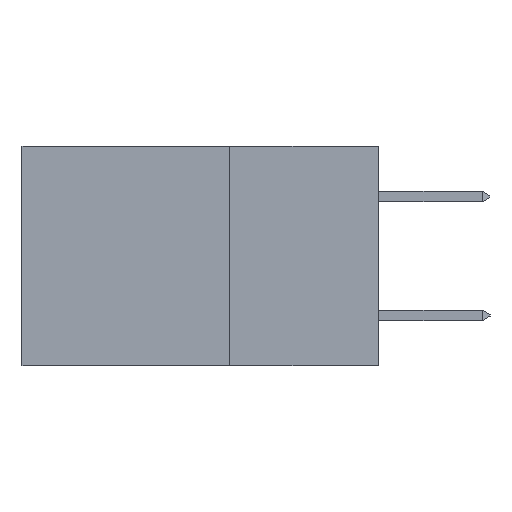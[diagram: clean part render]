
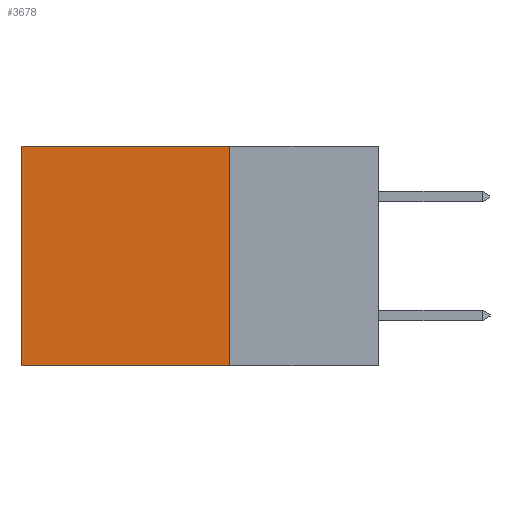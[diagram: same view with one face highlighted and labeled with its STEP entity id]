
A CAD part, left-side view. The second image highlights one B-rep face of the part: STEP entity #3678.
In plain terms, the highlighted planar face has unit normal (-1, 0, 0).
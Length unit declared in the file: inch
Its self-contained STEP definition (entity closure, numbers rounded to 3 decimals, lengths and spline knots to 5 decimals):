
#408 = VERTEX_POINT ( 'NONE', #5674 ) ;
#732 = VERTEX_POINT ( 'NONE', #3483 ) ;
#776 = DIRECTION ( 'NONE',  ( 0., 0., -1. ) ) ;
#1449 = ORIENTED_EDGE ( 'NONE', *, *, #1656, .F. ) ;
#1581 = VECTOR ( 'NONE', #10185, 39.37008 ) ;
#1656 = EDGE_CURVE ( 'NONE', #408, #4252, #3957, .T. ) ;
#1859 = CARTESIAN_POINT ( 'NONE',  ( 0.2615, 0.25, -0.37 ) ) ;
#1880 = VERTEX_POINT ( 'NONE', #9168 ) ;
#1961 = VECTOR ( 'NONE', #7360, 39.37008 ) ;
#2216 = DIRECTION ( 'NONE',  ( 1., 0., 0. ) ) ;
#2349 = EDGE_LOOP ( 'NONE', ( #9094, #3860, #1449, #4312 ) ) ;
#2393 = EDGE_CURVE ( 'NONE', #408, #1880, #5468, .T. ) ;
#3005 = CARTESIAN_POINT ( 'NONE',  ( 0.2615, 0.25, -0.37 ) ) ;
#3154 = FACE_OUTER_BOUND ( 'NONE', #2349, .T. ) ;
#3483 = CARTESIAN_POINT ( 'NONE',  ( 0.2615, 0.6, -0.37 ) ) ;
#3678 = ADVANCED_FACE ( 'NONE', ( #3154 ), #7095, .F. ) ;
#3860 = ORIENTED_EDGE ( 'NONE', *, *, #6834, .F. ) ;
#3957 = LINE ( 'NONE', #6675, #8181 ) ;
#4180 = CARTESIAN_POINT ( 'NONE',  ( 0.2615, 0.25, -0.37 ) ) ;
#4252 = VERTEX_POINT ( 'NONE', #1859 ) ;
#4312 = ORIENTED_EDGE ( 'NONE', *, *, #2393, .T. ) ;
#5369 = CARTESIAN_POINT ( 'NONE',  ( 0.2615, 0.25, 0. ) ) ;
#5468 = LINE ( 'NONE', #5369, #9268 ) ;
#5674 = CARTESIAN_POINT ( 'NONE',  ( 0.2615, 0.25, 0. ) ) ;
#6159 = AXIS2_PLACEMENT_3D ( 'NONE', #3005, #2216, #7846 ) ;
#6347 = LINE ( 'NONE', #6593, #1961 ) ;
#6593 = CARTESIAN_POINT ( 'NONE',  ( 0.2615, 0.6, -0.37 ) ) ;
#6675 = CARTESIAN_POINT ( 'NONE',  ( 0.2615, 0.25, -0.37 ) ) ;
#6834 = EDGE_CURVE ( 'NONE', #4252, #732, #8047, .T. ) ;
#7095 = PLANE ( 'NONE',  #6159 ) ;
#7360 = DIRECTION ( 'NONE',  ( 0., 0., -1. ) ) ;
#7846 = DIRECTION ( 'NONE',  ( 0., 0., -1. ) ) ;
#8047 = LINE ( 'NONE', #4180, #1581 ) ;
#8181 = VECTOR ( 'NONE', #776, 39.37008 ) ;
#9094 = ORIENTED_EDGE ( 'NONE', *, *, #9296, .T. ) ;
#9168 = CARTESIAN_POINT ( 'NONE',  ( 0.2615, 0.6, 0. ) ) ;
#9268 = VECTOR ( 'NONE', #9848, 39.37008 ) ;
#9296 = EDGE_CURVE ( 'NONE', #1880, #732, #6347, .T. ) ;
#9848 = DIRECTION ( 'NONE',  ( 0., 1., 0. ) ) ;
#10185 = DIRECTION ( 'NONE',  ( 0., 1., 0. ) ) ;
